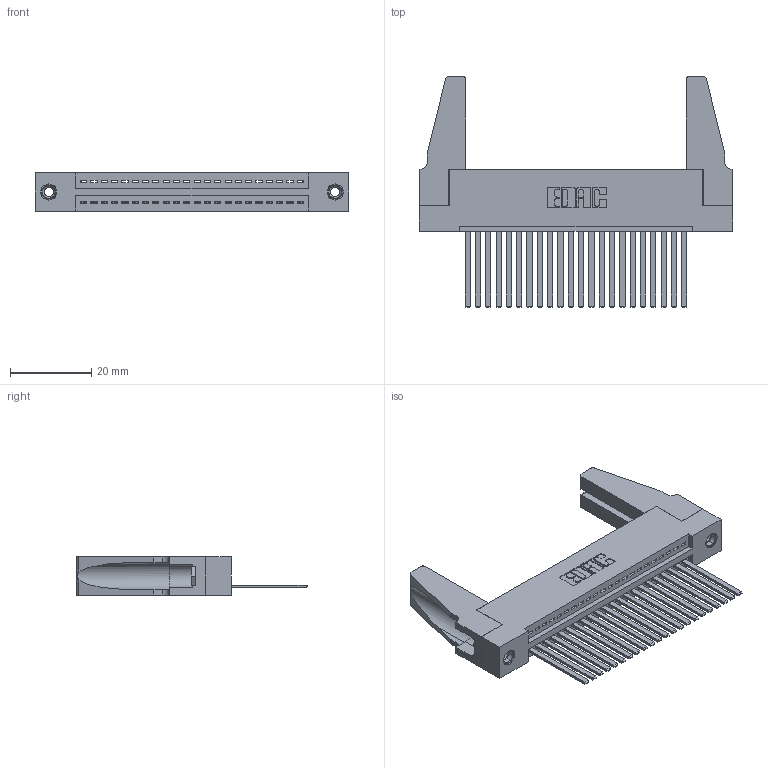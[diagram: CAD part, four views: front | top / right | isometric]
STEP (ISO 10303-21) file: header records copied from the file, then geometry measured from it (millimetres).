
FILE_DESCRIPTION (( 'STEP AP203' ), '1' );
FILE_NAME ('345-022-544-188.STEP', '2019-10-05T00:56:42', ( '' ), ( '' ), 'SwSTEP 2.0', 'SolidWorks 2016', '' );
FILE_SCHEMA (( 'CONFIG_CONTROL_DESIGN' ));
Length unit declared in the file: inch
Products named in the file (5): 345 Part_Flush Mounting Lugs - 0.156 Dia-TH; 345-292-001_345-293-144; 345-220-078_345-220-088; 345-250-001_345-250-001-102; 345-022-544-188
Assembly tree (27 placements, depth 2):
  345-022-544-188
    345 Part_Flush Mounting Lugs - 0.156 Dia-TH
    345-292-001_345-293-144  x22
    345-250-001_345-250-001-102  x2
    345-220-078_345-220-088  x2
Bounding box: 77.11 x 56.82 x 9.4 mm (x, y, z)
Volume: 10667.9 mm3; surface area: 13476.7 mm2
Topology: 27 solids, 27 shells, 1394 faces, 4131 edges, 2714 vertices
Faces by surface type: plane 944, cylinder 434, cone 12, torus 4
Entity records: 21214 total; most frequent: CARTESIAN_POINT 3664, ORIENTED_EDGE 3580, DIRECTION 3234, EDGE_CURVE 1790, VECTOR 1532, LINE 1532, VERTEX_POINT 1186, AXIS2_PLACEMENT_3D 851
